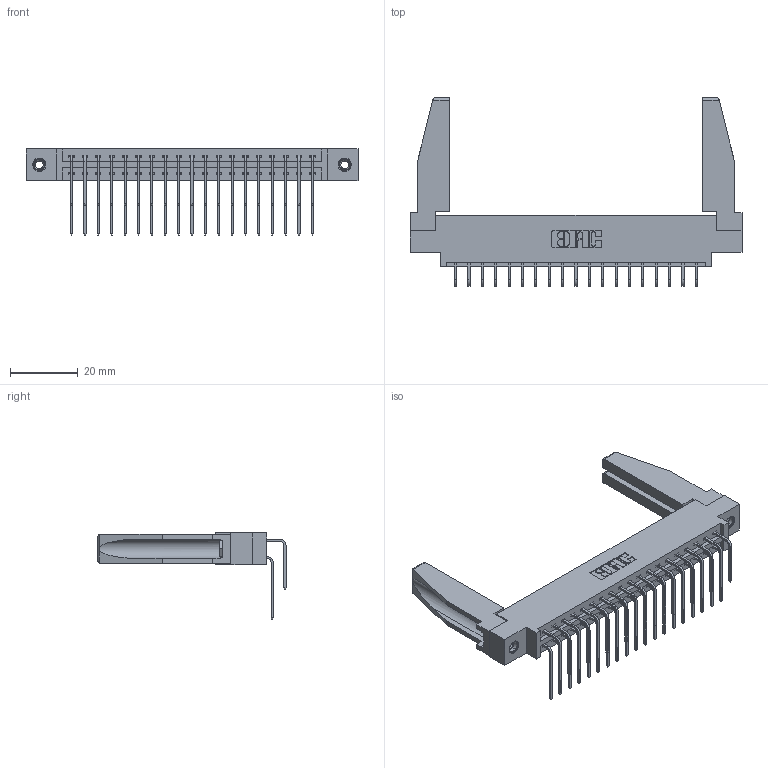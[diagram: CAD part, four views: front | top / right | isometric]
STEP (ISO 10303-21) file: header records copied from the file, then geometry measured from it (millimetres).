
FILE_DESCRIPTION (( 'STEP AP203' ), '1' );
FILE_NAME ('337-038-559-878.STEP', '2019-10-11T11:43:02', ( '' ), ( '' ), 'SwSTEP 2.0', 'SolidWorks 2016', '' );
FILE_SCHEMA (( 'CONFIG_CONTROL_DESIGN' ));
Length unit declared in the file: inch
Products named in the file (6): 345-292-001_559 Tail - 2; 345-292-001_558 559 Tail - 1; 307-220-078; 345-250-001_345-250-001-102; 337 Part_0.170 Offset - 0.156 Dia-TI; 337-038-559-878
Assembly tree (43 placements, depth 2):
  337-038-559-878
    337 Part_0.170 Offset - 0.156 Dia-TI
    345-292-001_558 559 Tail - 1  x19
    345-292-001_559 Tail - 2  x19
    345-250-001_345-250-001-102  x2
    307-220-078  x2
Bounding box: 98.3 x 55.69 x 25.53 mm (x, y, z)
Volume: 14148.3 mm3; surface area: 16295.8 mm2
Topology: 43 solids, 43 shells, 2376 faces, 6999 edges, 4606 vertices
Faces by surface type: plane 1678, cylinder 682, cone 12, torus 4
Entity records: 22062 total; most frequent: CARTESIAN_POINT 3783, ORIENTED_EDGE 3624, DIRECTION 3248, EDGE_CURVE 1812, LINE 1606, VECTOR 1606, VERTEX_POINT 1200, AXIS2_PLACEMENT_3D 821
